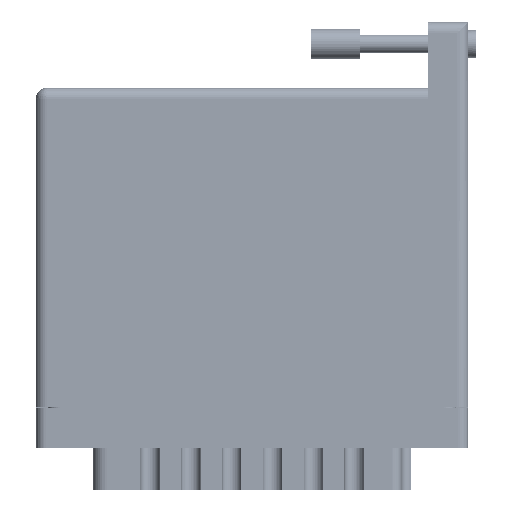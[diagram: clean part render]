
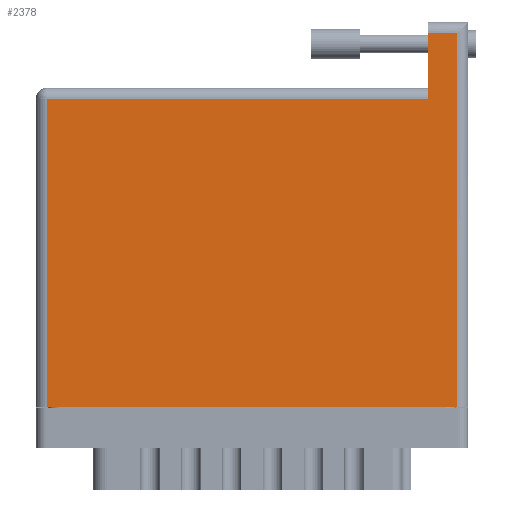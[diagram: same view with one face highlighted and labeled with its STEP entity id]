
A CAD part, front view. The second image highlights one B-rep face of the part: STEP entity #2378.
In plain terms, the highlighted face is planar.
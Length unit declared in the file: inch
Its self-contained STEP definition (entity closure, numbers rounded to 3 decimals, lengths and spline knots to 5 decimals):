
#1500 = VERTEX_POINT ( 'NONE', #41110 ) ;
#1681 = VECTOR ( 'NONE', #18174, 39.37008 ) ;
#2027 = DIRECTION ( 'NONE',  ( 0., 0., -1. ) ) ;
#2272 = VERTEX_POINT ( 'NONE', #52306 ) ;
#2293 = AXIS2_PLACEMENT_3D ( 'NONE', #17047, #2027, #9867 ) ;
#2378 = ADVANCED_FACE ( 'NONE', ( #70341 ), #54545, .F. ) ;
#3961 = CARTESIAN_POINT ( 'NONE',  ( 2.685, 0., 0. ) ) ;
#6075 = EDGE_CURVE ( 'NONE', #67554, #1500, #10957, .T. ) ;
#7150 = LINE ( 'NONE', #53422, #68966 ) ;
#9867 = DIRECTION ( 'NONE',  ( -1., 0., 0. ) ) ;
#10957 = LINE ( 'NONE', #51822, #49551 ) ;
#11591 = DIRECTION ( 'NONE',  ( 1., 0., 0. ) ) ;
#17047 = CARTESIAN_POINT ( 'NONE',  ( 0., 2.03, 0. ) ) ;
#17977 = CARTESIAN_POINT ( 'NONE',  ( 2.685, 2.45, 0. ) ) ;
#18174 = DIRECTION ( 'NONE',  ( 0., -1., 0. ) ) ;
#20585 = LINE ( 'NONE', #72200, #75355 ) ;
#26071 = ORIENTED_EDGE ( 'NONE', *, *, #48460, .T. ) ;
#28063 = ORIENTED_EDGE ( 'NONE', *, *, #64608, .T. ) ;
#28691 = VERTEX_POINT ( 'NONE', #86663 ) ;
#28748 = ORIENTED_EDGE ( 'NONE', *, *, #47636, .T. ) ;
#28932 = LINE ( 'NONE', #17977, #60386 ) ;
#29869 = EDGE_CURVE ( 'NONE', #71746, #95578, #55691, .T. ) ;
#36705 = ORIENTED_EDGE ( 'NONE', *, *, #29869, .T. ) ;
#41110 = CARTESIAN_POINT ( 'NONE',  ( 2.499, 2.38, 0. ) ) ;
#47607 = VECTOR ( 'NONE', #11591, 39.37008 ) ;
#47636 = EDGE_CURVE ( 'NONE', #95578, #67554, #28932, .T. ) ;
#48460 = EDGE_CURVE ( 'NONE', #1500, #2272, #20585, .T. ) ;
#49260 = EDGE_LOOP ( 'NONE', ( #26071, #28063, #93821, #36705, #28748, #49434 ) ) ;
#49434 = ORIENTED_EDGE ( 'NONE', *, *, #6075, .T. ) ;
#49551 = VECTOR ( 'NONE', #66687, 39.37008 ) ;
#49787 = DIRECTION ( 'NONE',  ( 0., -1., 0. ) ) ;
#51822 = CARTESIAN_POINT ( 'NONE',  ( 0., 2.38, 0. ) ) ;
#52306 = CARTESIAN_POINT ( 'NONE',  ( 2.499, 1.96, 0. ) ) ;
#53422 = CARTESIAN_POINT ( 'NONE',  ( 0., 1.96, 0. ) ) ;
#54059 = DIRECTION ( 'NONE',  ( -1., 0., 0. ) ) ;
#54545 = PLANE ( 'NONE',  #2293 ) ;
#55339 = CARTESIAN_POINT ( 'NONE',  ( 0.07, 0., 0. ) ) ;
#55691 = LINE ( 'NONE', #85816, #47607 ) ;
#55768 = DIRECTION ( 'NONE',  ( 0., 1., 0. ) ) ;
#60386 = VECTOR ( 'NONE', #55768, 39.37008 ) ;
#64608 = EDGE_CURVE ( 'NONE', #2272, #28691, #7150, .T. ) ;
#64672 = LINE ( 'NONE', #55339, #1681 ) ;
#66687 = DIRECTION ( 'NONE',  ( -1., 0., 0. ) ) ;
#67554 = VERTEX_POINT ( 'NONE', #93683 ) ;
#68966 = VECTOR ( 'NONE', #54059, 39.37008 ) ;
#70341 = FACE_OUTER_BOUND ( 'NONE', #49260, .T. ) ;
#71746 = VERTEX_POINT ( 'NONE', #94895 ) ;
#72200 = CARTESIAN_POINT ( 'NONE',  ( 2.499, 2.45, 0. ) ) ;
#75355 = VECTOR ( 'NONE', #49787, 39.37008 ) ;
#85816 = CARTESIAN_POINT ( 'NONE',  ( 0., 0., 0. ) ) ;
#86663 = CARTESIAN_POINT ( 'NONE',  ( 0.07, 1.96, 0. ) ) ;
#87520 = EDGE_CURVE ( 'NONE', #28691, #71746, #64672, .T. ) ;
#93683 = CARTESIAN_POINT ( 'NONE',  ( 2.685, 2.38, 0. ) ) ;
#93821 = ORIENTED_EDGE ( 'NONE', *, *, #87520, .T. ) ;
#94895 = CARTESIAN_POINT ( 'NONE',  ( 0.07, 0., 0. ) ) ;
#95578 = VERTEX_POINT ( 'NONE', #3961 ) ;
